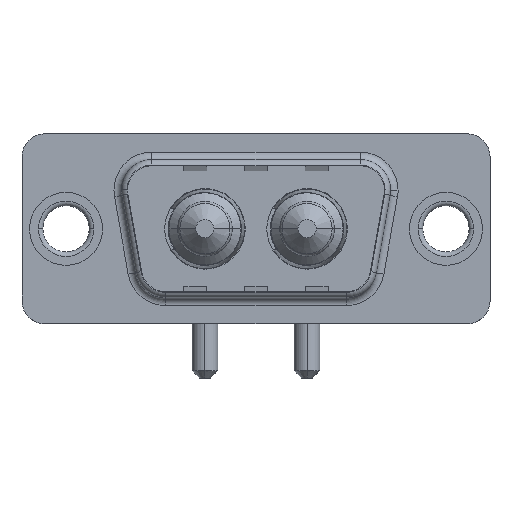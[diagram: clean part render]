
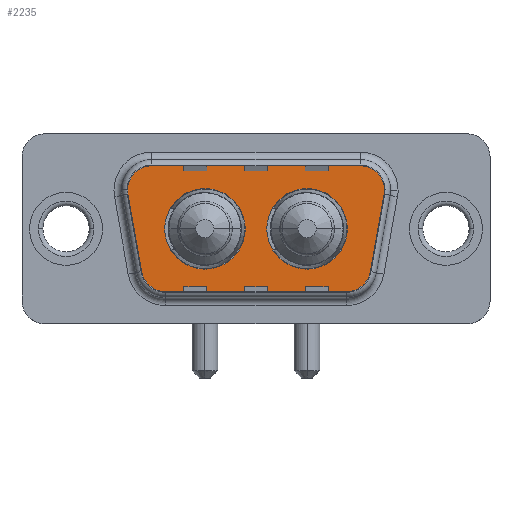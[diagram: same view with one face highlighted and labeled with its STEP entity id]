
A CAD part, top view. The second image highlights one B-rep face of the part: STEP entity #2235.
In plain terms, the highlighted planar face has unit normal (0, 0, 1).
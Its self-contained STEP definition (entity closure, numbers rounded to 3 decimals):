
#297 = CARTESIAN_POINT ( 'NONE',  ( 18.51, 0., 0. ) ) ;
#332 = DIRECTION ( 'NONE',  ( 0., 0., 1. ) ) ;
#396 = DIRECTION ( 'NONE',  ( 0., 0., 1. ) ) ;
#400 = DIRECTION ( 'NONE',  ( -1., 0., 0. ) ) ;
#442 = DIRECTION ( 'NONE',  ( 0.174, 0.985, 0. ) ) ;
#448 = DIRECTION ( 'NONE',  ( 1., 0., 0. ) ) ;
#646 = VECTOR ( 'NONE', #2224, 1000. ) ;
#766 = AXIS2_PLACEMENT_3D ( 'NONE', #4402, #9630, #448 ) ;
#770 = VECTOR ( 'NONE', #8445, 1000. ) ;
#780 = EDGE_CURVE ( 'NONE', #3658, #5599, #8576, .T. ) ;
#815 = CIRCLE ( 'NONE', #6324, 2. ) ;
#839 = DIRECTION ( 'NONE',  ( 0., 0., 1. ) ) ;
#909 = CARTESIAN_POINT ( 'NONE',  ( 18.541, -2.9, 0. ) ) ;
#1060 = DIRECTION ( 'NONE',  ( 0., 0., 1. ) ) ;
#1099 = CARTESIAN_POINT ( 'NONE',  ( 5.436, 2.9, 0. ) ) ;
#1535 = VERTEX_POINT ( 'NONE', #7197 ) ;
#1602 = DIRECTION ( 'NONE',  ( 0., 0., 1. ) ) ;
#1640 = ORIENTED_EDGE ( 'NONE', *, *, #4345, .F. ) ;
#1653 = FACE_BOUND ( 'NONE', #5288, .T. ) ;
#1729 = ORIENTED_EDGE ( 'NONE', *, *, #6958, .T. ) ;
#1927 = ORIENTED_EDGE ( 'NONE', *, *, #9298, .T. ) ;
#2023 = LINE ( 'NONE', #4305, #5030 ) ;
#2097 = AXIS2_PLACEMENT_3D ( 'NONE', #6950, #332, #6153 ) ;
#2169 = VERTEX_POINT ( 'NONE', #3166 ) ;
#2224 = DIRECTION ( 'NONE',  ( -1., 0., 0. ) ) ;
#2235 = ADVANCED_FACE ( 'NONE', ( #9139, #1653, #3075 ), #7770, .T. ) ;
#2241 = CARTESIAN_POINT ( 'NONE',  ( 13.21, 0., 0. ) ) ;
#2275 = CARTESIAN_POINT ( 'NONE',  ( 6.459, -4.9, 0. ) ) ;
#2511 = VERTEX_POINT ( 'NONE', #2241 ) ;
#2515 = AXIS2_PLACEMENT_3D ( 'NONE', #4098, #7164, #400 ) ;
#2719 = ORIENTED_EDGE ( 'NONE', *, *, #2895, .T. ) ;
#2836 = VERTEX_POINT ( 'NONE', #297 ) ;
#2895 = EDGE_CURVE ( 'NONE', #2169, #9513, #5679, .T. ) ;
#2901 = EDGE_CURVE ( 'NONE', #9513, #3658, #8788, .T. ) ;
#2998 = AXIS2_PLACEMENT_3D ( 'NONE', #7880, #839, #6871 ) ;
#3075 = FACE_OUTER_BOUND ( 'NONE', #3376, .T. ) ;
#3092 = LINE ( 'NONE', #2275, #9344 ) ;
#3106 = EDGE_CURVE ( 'NONE', #4288, #1535, #3470, .T. ) ;
#3166 = CARTESIAN_POINT ( 'NONE',  ( 21.564, 2.9, 0. ) ) ;
#3169 = AXIS2_PLACEMENT_3D ( 'NONE', #909, #4016, #4617 ) ;
#3335 = DIRECTION ( 'NONE',  ( 1., 0., 0. ) ) ;
#3376 = EDGE_LOOP ( 'NONE', ( #8309, #1729, #3413, #2719, #6776, #6137, #8536, #5585, #1927 ) ) ;
#3398 = DIRECTION ( 'NONE',  ( -1., 0., 0. ) ) ;
#3413 = ORIENTED_EDGE ( 'NONE', *, *, #7719, .T. ) ;
#3460 = AXIS2_PLACEMENT_3D ( 'NONE', #6893, #1602, #3870 ) ;
#3470 = CIRCLE ( 'NONE', #2998, 2.65 ) ;
#3529 = EDGE_CURVE ( 'NONE', #6075, #7795, #3634, .T. ) ;
#3634 = CIRCLE ( 'NONE', #3460, 2. ) ;
#3635 = EDGE_CURVE ( 'NONE', #3687, #8254, #8680, .T. ) ;
#3658 = VERTEX_POINT ( 'NONE', #4567 ) ;
#3687 = VERTEX_POINT ( 'NONE', #9438 ) ;
#3751 = ORIENTED_EDGE ( 'NONE', *, *, #5004, .F. ) ;
#3870 = DIRECTION ( 'NONE',  ( 1., 0., 0. ) ) ;
#4016 = DIRECTION ( 'NONE',  ( 0., 0., 1. ) ) ;
#4098 = CARTESIAN_POINT ( 'NONE',  ( 19.564, 2.9, 0. ) ) ;
#4288 = VERTEX_POINT ( 'NONE', #8149 ) ;
#4305 = CARTESIAN_POINT ( 'NONE',  ( 21.534, 2.553, 0. ) ) ;
#4345 = EDGE_CURVE ( 'NONE', #2511, #2836, #4856, .T. ) ;
#4402 = CARTESIAN_POINT ( 'NONE',  ( 15.86, 0., 0. ) ) ;
#4567 = CARTESIAN_POINT ( 'NONE',  ( 5.436, 4.9, 0. ) ) ;
#4617 = DIRECTION ( 'NONE',  ( 1., 0., 0. ) ) ;
#4637 = VERTEX_POINT ( 'NONE', #9261 ) ;
#4856 = CIRCLE ( 'NONE', #766, 2.65 ) ;
#4889 = CARTESIAN_POINT ( 'NONE',  ( 19.564, 2.9, 0. ) ) ;
#4900 = ORIENTED_EDGE ( 'NONE', *, *, #5017, .F. ) ;
#5004 = EDGE_CURVE ( 'NONE', #1535, #4288, #8718, .T. ) ;
#5017 = EDGE_CURVE ( 'NONE', #2836, #2511, #8249, .T. ) ;
#5024 = CARTESIAN_POINT ( 'NONE',  ( 18.541, -4.9, 0. ) ) ;
#5030 = VECTOR ( 'NONE', #442, 1000. ) ;
#5288 = EDGE_LOOP ( 'NONE', ( #5940, #3751 ) ) ;
#5345 = DIRECTION ( 'NONE',  ( 0., 0., 1. ) ) ;
#5585 = ORIENTED_EDGE ( 'NONE', *, *, #3635, .T. ) ;
#5599 = VERTEX_POINT ( 'NONE', #7948 ) ;
#5679 = CIRCLE ( 'NONE', #2515, 2. ) ;
#5879 = CARTESIAN_POINT ( 'NONE',  ( 5.436, 4.9, 0. ) ) ;
#5940 = ORIENTED_EDGE ( 'NONE', *, *, #3106, .F. ) ;
#5965 = DIRECTION ( 'NONE',  ( 1., 0., 0. ) ) ;
#6075 = VERTEX_POINT ( 'NONE', #5024 ) ;
#6137 = ORIENTED_EDGE ( 'NONE', *, *, #780, .T. ) ;
#6153 = DIRECTION ( 'NONE',  ( 1., 0., 0. ) ) ;
#6168 = LINE ( 'NONE', #9180, #770 ) ;
#6185 = AXIS2_PLACEMENT_3D ( 'NONE', #9160, #1060, #3335 ) ;
#6324 = AXIS2_PLACEMENT_3D ( 'NONE', #4889, #396, #3398 ) ;
#6387 = DIRECTION ( 'NONE',  ( 0., 0., 1. ) ) ;
#6776 = ORIENTED_EDGE ( 'NONE', *, *, #2901, .T. ) ;
#6847 = EDGE_CURVE ( 'NONE', #5599, #3687, #6168, .T. ) ;
#6871 = DIRECTION ( 'NONE',  ( 1., 0., 0. ) ) ;
#6893 = CARTESIAN_POINT ( 'NONE',  ( 18.541, -2.9, 0. ) ) ;
#6948 = AXIS2_PLACEMENT_3D ( 'NONE', #8418, #5345, #9145 ) ;
#6950 = CARTESIAN_POINT ( 'NONE',  ( 9.14, 0., 0. ) ) ;
#6958 = EDGE_CURVE ( 'NONE', #7795, #4637, #2023, .T. ) ;
#7136 = DIRECTION ( 'NONE',  ( 1., 0., 0. ) ) ;
#7164 = DIRECTION ( 'NONE',  ( 0., 0., 1. ) ) ;
#7197 = CARTESIAN_POINT ( 'NONE',  ( 6.49, 0., 0. ) ) ;
#7377 = CARTESIAN_POINT ( 'NONE',  ( 6.459, -4.9, 0. ) ) ;
#7394 = CARTESIAN_POINT ( 'NONE',  ( 19.564, 4.9, 0. ) ) ;
#7401 = CARTESIAN_POINT ( 'NONE',  ( 20.511, -3.247, 0. ) ) ;
#7719 = EDGE_CURVE ( 'NONE', #4637, #2169, #815, .T. ) ;
#7770 = PLANE ( 'NONE',  #3169 ) ;
#7795 = VERTEX_POINT ( 'NONE', #7401 ) ;
#7880 = CARTESIAN_POINT ( 'NONE',  ( 9.14, 0., 0. ) ) ;
#7948 = CARTESIAN_POINT ( 'NONE',  ( 3.466, 2.553, 0. ) ) ;
#8149 = CARTESIAN_POINT ( 'NONE',  ( 11.79, 0., 0. ) ) ;
#8249 = CIRCLE ( 'NONE', #6185, 2.65 ) ;
#8254 = VERTEX_POINT ( 'NONE', #7377 ) ;
#8273 = AXIS2_PLACEMENT_3D ( 'NONE', #1099, #6387, #7136 ) ;
#8309 = ORIENTED_EDGE ( 'NONE', *, *, #3529, .T. ) ;
#8418 = CARTESIAN_POINT ( 'NONE',  ( 6.459, -2.9, 0. ) ) ;
#8445 = DIRECTION ( 'NONE',  ( 0.174, -0.985, 0. ) ) ;
#8536 = ORIENTED_EDGE ( 'NONE', *, *, #6847, .T. ) ;
#8576 = CIRCLE ( 'NONE', #8273, 2. ) ;
#8680 = CIRCLE ( 'NONE', #6948, 2. ) ;
#8718 = CIRCLE ( 'NONE', #2097, 2.65 ) ;
#8788 = LINE ( 'NONE', #5879, #646 ) ;
#9139 = FACE_BOUND ( 'NONE', #9359, .T. ) ;
#9145 = DIRECTION ( 'NONE',  ( -1., 0., 0. ) ) ;
#9160 = CARTESIAN_POINT ( 'NONE',  ( 15.86, 0., 0. ) ) ;
#9180 = CARTESIAN_POINT ( 'NONE',  ( 3.466, 2.553, 0. ) ) ;
#9261 = CARTESIAN_POINT ( 'NONE',  ( 21.534, 2.553, 0. ) ) ;
#9298 = EDGE_CURVE ( 'NONE', #8254, #6075, #3092, .T. ) ;
#9344 = VECTOR ( 'NONE', #5965, 1000. ) ;
#9359 = EDGE_LOOP ( 'NONE', ( #4900, #1640 ) ) ;
#9438 = CARTESIAN_POINT ( 'NONE',  ( 4.489, -3.247, 0. ) ) ;
#9513 = VERTEX_POINT ( 'NONE', #7394 ) ;
#9630 = DIRECTION ( 'NONE',  ( 0., 0., 1. ) ) ;
